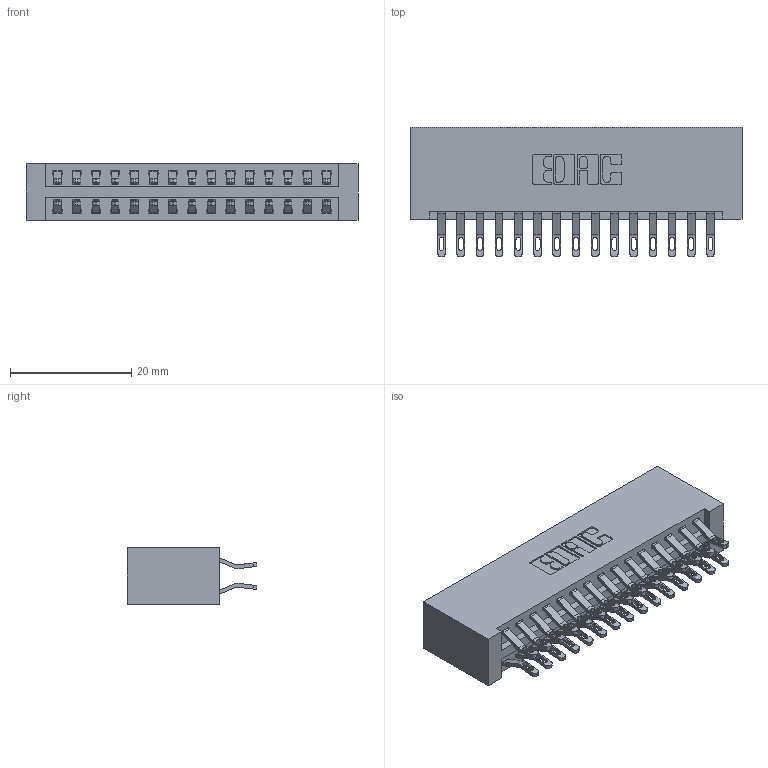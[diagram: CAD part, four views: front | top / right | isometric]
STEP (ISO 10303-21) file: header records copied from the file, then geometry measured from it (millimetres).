
FILE_DESCRIPTION (( 'STEP AP203' ), '1' );
FILE_NAME ('346-030-555-201.STEP', '2022-05-19T16:42:02', ( '' ), ( '' ), 'SwSTEP 2.0', 'SolidWorks 2020', '' );
FILE_SCHEMA (( 'CONFIG_CONTROL_DESIGN' ));
Length unit declared in the file: inch
Products named in the file (3): 345-292-001_555 Tail; 346 Part_No Mounting Lugs; 346-030-555-201
Assembly tree (31 placements, depth 2):
  346-030-555-201
    346 Part_No Mounting Lugs
    345-292-001_555 Tail  x30
Bounding box: 54.86 x 21.46 x 9.4 mm (x, y, z)
Volume: 5800.5 mm3; surface area: 8022.2 mm2
Topology: 31 solids, 31 shells, 1854 faces, 5795 edges, 3862 vertices
Faces by surface type: plane 1062, cylinder 792
Entity records: 13473 total; most frequent: CARTESIAN_POINT 2290, ORIENTED_EDGE 2194, DIRECTION 2033, EDGE_CURVE 1097, VECTOR 893, LINE 893, VERTEX_POINT 730, AXIS2_PLACEMENT_3D 570
